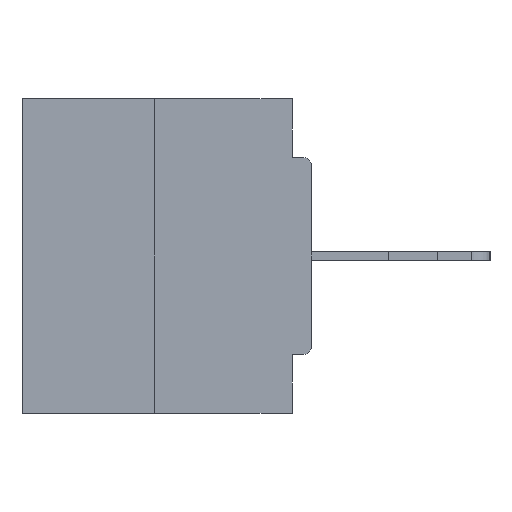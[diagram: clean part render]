
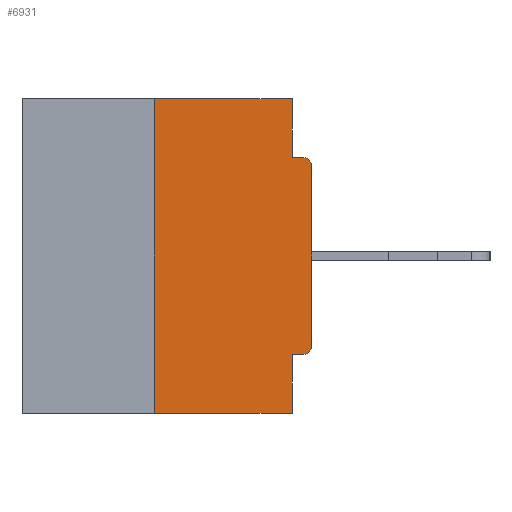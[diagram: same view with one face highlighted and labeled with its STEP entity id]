
A CAD part, left-side view. The second image highlights one B-rep face of the part: STEP entity #6931.
In plain terms, the highlighted planar face has unit normal (-1, 0, 0).
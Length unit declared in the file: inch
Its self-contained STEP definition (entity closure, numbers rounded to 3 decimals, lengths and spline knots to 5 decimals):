
#72 = LINE ( 'NONE', #12369, #28594 ) ;
#321 = CARTESIAN_POINT ( 'NONE',  ( 0., 0., -0.4065 ) ) ;
#655 = DIRECTION ( 'NONE',  ( 0., 1., 0. ) ) ;
#1202 = LINE ( 'NONE', #32012, #11351 ) ;
#1540 = EDGE_LOOP ( 'NONE', ( #2131, #5607, #6579, #12016, #21426, #31265, #19724, #21570, #19228, #2540 ) ) ;
#1609 = DIRECTION ( 'NONE',  ( 0., 0., -1. ) ) ;
#1710 = DIRECTION ( 'NONE',  ( 0., 0., 1. ) ) ;
#2131 = ORIENTED_EDGE ( 'NONE', *, *, #27432, .F. ) ;
#2540 = ORIENTED_EDGE ( 'NONE', *, *, #25512, .F. ) ;
#4606 = CARTESIAN_POINT ( 'NONE',  ( 0., 0.015, -0.3915 ) ) ;
#4792 = AXIS2_PLACEMENT_3D ( 'NONE', #4606, #6641, #1609 ) ;
#5486 = CARTESIAN_POINT ( 'NONE',  ( 0., 0.015, -0.0935 ) ) ;
#5607 = ORIENTED_EDGE ( 'NONE', *, *, #14384, .F. ) ;
#6579 = ORIENTED_EDGE ( 'NONE', *, *, #24890, .T. ) ;
#6641 = DIRECTION ( 'NONE',  ( -1., 0., 0. ) ) ;
#6727 = DIRECTION ( 'NONE',  ( -1., 0., 0. ) ) ;
#6777 = EDGE_CURVE ( 'NONE', #18457, #10555, #1202, .T. ) ;
#6931 = ADVANCED_FACE ( 'NONE', ( #12624 ), #22888, .F. ) ;
#7402 = CARTESIAN_POINT ( 'NONE',  ( 0., 0.46, 0. ) ) ;
#7461 = VECTOR ( 'NONE', #655, 39.37008 ) ;
#7890 = CARTESIAN_POINT ( 'NONE',  ( 0., 0., -0.0935 ) ) ;
#8224 = LINE ( 'NONE', #7890, #28054 ) ;
#9514 = CIRCLE ( 'NONE', #27291, 0.015 ) ;
#9756 = DIRECTION ( 'NONE',  ( 0., 0., -1. ) ) ;
#10555 = VERTEX_POINT ( 'NONE', #26561 ) ;
#10924 = DIRECTION ( 'NONE',  ( 0., -1., 0. ) ) ;
#11321 = VECTOR ( 'NONE', #33056, 39.37008 ) ;
#11337 = VERTEX_POINT ( 'NONE', #13630 ) ;
#11351 = VECTOR ( 'NONE', #1710, 39.37008 ) ;
#11623 = CARTESIAN_POINT ( 'NONE',  ( 0., 0.015, -0.1085 ) ) ;
#12016 = ORIENTED_EDGE ( 'NONE', *, *, #32965, .F. ) ;
#12113 = DIRECTION ( 'NONE',  ( 0., -1., 0. ) ) ;
#12238 = CARTESIAN_POINT ( 'NONE',  ( 0., 0.031, 0. ) ) ;
#12369 = CARTESIAN_POINT ( 'NONE',  ( 0., 0.031, -0.5 ) ) ;
#12624 = FACE_OUTER_BOUND ( 'NONE', #1540, .T. ) ;
#12875 = CARTESIAN_POINT ( 'NONE',  ( 0., 0.031, 0. ) ) ;
#13204 = DIRECTION ( 'NONE',  ( 0., 0., -1. ) ) ;
#13630 = CARTESIAN_POINT ( 'NONE',  ( 0., 0.031, -0.0935 ) ) ;
#14128 = CARTESIAN_POINT ( 'NONE',  ( 0., 0.46, -0.5 ) ) ;
#14384 = EDGE_CURVE ( 'NONE', #23200, #24619, #18128, .T. ) ;
#16727 = VERTEX_POINT ( 'NONE', #12238 ) ;
#17024 = VERTEX_POINT ( 'NONE', #21132 ) ;
#17552 = CARTESIAN_POINT ( 'NONE',  ( 0., 0.25, -0.5 ) ) ;
#17850 = CARTESIAN_POINT ( 'NONE',  ( 0., 0.25, 0. ) ) ;
#18002 = DIRECTION ( 'NONE',  ( 1., 0., 0. ) ) ;
#18109 = VERTEX_POINT ( 'NONE', #5486 ) ;
#18128 = LINE ( 'NONE', #23182, #25577 ) ;
#18457 = VERTEX_POINT ( 'NONE', #30897 ) ;
#19228 = ORIENTED_EDGE ( 'NONE', *, *, #28192, .F. ) ;
#19525 = LINE ( 'NONE', #14128, #26768 ) ;
#19714 = VERTEX_POINT ( 'NONE', #32311 ) ;
#19724 = ORIENTED_EDGE ( 'NONE', *, *, #6777, .T. ) ;
#21132 = CARTESIAN_POINT ( 'NONE',  ( 0., 0.015, -0.4065 ) ) ;
#21426 = ORIENTED_EDGE ( 'NONE', *, *, #31125, .F. ) ;
#21570 = ORIENTED_EDGE ( 'NONE', *, *, #23643, .T. ) ;
#21571 = EDGE_CURVE ( 'NONE', #17024, #18457, #31722, .T. ) ;
#22639 = DIRECTION ( 'NONE',  ( 0., 0., -1. ) ) ;
#22888 = PLANE ( 'NONE',  #27506 ) ;
#23182 = CARTESIAN_POINT ( 'NONE',  ( 0., 0.25, 0. ) ) ;
#23200 = VERTEX_POINT ( 'NONE', #17552 ) ;
#23643 = EDGE_CURVE ( 'NONE', #10555, #18109, #9514, .T. ) ;
#24619 = VERTEX_POINT ( 'NONE', #17850 ) ;
#24676 = VECTOR ( 'NONE', #13204, 39.37008 ) ;
#24890 = EDGE_CURVE ( 'NONE', #23200, #19714, #19525, .T. ) ;
#24921 = CARTESIAN_POINT ( 'NONE',  ( 0., 0.031, -0.4065 ) ) ;
#25275 = LINE ( 'NONE', #7402, #11321 ) ;
#25386 = DIRECTION ( 'NONE',  ( 0., 0., 1. ) ) ;
#25512 = EDGE_CURVE ( 'NONE', #16727, #11337, #25680, .T. ) ;
#25577 = VECTOR ( 'NONE', #25386, 39.37008 ) ;
#25680 = LINE ( 'NONE', #12875, #24676 ) ;
#26192 = VERTEX_POINT ( 'NONE', #24921 ) ;
#26404 = LINE ( 'NONE', #321, #7461 ) ;
#26561 = CARTESIAN_POINT ( 'NONE',  ( 0., 0., -0.1085 ) ) ;
#26768 = VECTOR ( 'NONE', #12113, 39.37008 ) ;
#27291 = AXIS2_PLACEMENT_3D ( 'NONE', #11623, #6727, #9756 ) ;
#27432 = EDGE_CURVE ( 'NONE', #24619, #16727, #25275, .T. ) ;
#27506 = AXIS2_PLACEMENT_3D ( 'NONE', #33184, #18002, #28308 ) ;
#28054 = VECTOR ( 'NONE', #10924, 39.37008 ) ;
#28192 = EDGE_CURVE ( 'NONE', #11337, #18109, #8224, .T. ) ;
#28308 = DIRECTION ( 'NONE',  ( 0., 0., -1. ) ) ;
#28594 = VECTOR ( 'NONE', #22639, 39.37008 ) ;
#30897 = CARTESIAN_POINT ( 'NONE',  ( 0., 0., -0.3915 ) ) ;
#31125 = EDGE_CURVE ( 'NONE', #17024, #26192, #26404, .T. ) ;
#31265 = ORIENTED_EDGE ( 'NONE', *, *, #21571, .T. ) ;
#31722 = CIRCLE ( 'NONE', #4792, 0.015 ) ;
#32012 = CARTESIAN_POINT ( 'NONE',  ( 0., 0., 0. ) ) ;
#32311 = CARTESIAN_POINT ( 'NONE',  ( 0., 0.031, -0.5 ) ) ;
#32965 = EDGE_CURVE ( 'NONE', #26192, #19714, #72, .T. ) ;
#33056 = DIRECTION ( 'NONE',  ( 0., -1., 0. ) ) ;
#33184 = CARTESIAN_POINT ( 'NONE',  ( 0., 0.46, 0. ) ) ;
